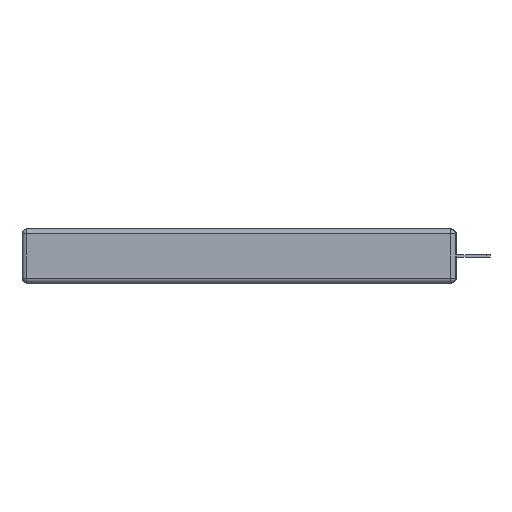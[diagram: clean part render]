
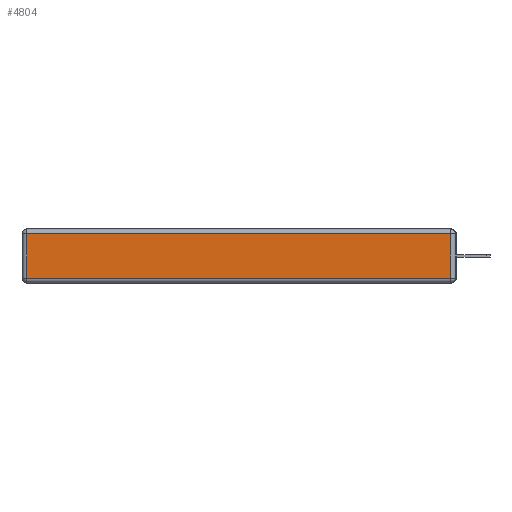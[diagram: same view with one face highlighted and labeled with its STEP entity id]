
A CAD part, left-side view. The second image highlights one B-rep face of the part: STEP entity #4804.
In plain terms, the highlighted planar face has unit normal (-1, 0, 0).
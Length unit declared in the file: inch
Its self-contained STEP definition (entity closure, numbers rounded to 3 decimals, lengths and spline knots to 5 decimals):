
#715 = EDGE_CURVE ( 'NONE', #19303, #4121, #13686, .T. ) ;
#1388 = VERTEX_POINT ( 'NONE', #10222 ) ;
#2633 = FACE_OUTER_BOUND ( 'NONE', #12897, .T. ) ;
#3143 = EDGE_CURVE ( 'NONE', #7421, #19303, #9139, .T. ) ;
#4050 = LINE ( 'NONE', #9018, #18800 ) ;
#4121 = VERTEX_POINT ( 'NONE', #5775 ) ;
#4445 = ORIENTED_EDGE ( 'NONE', *, *, #8056, .T. ) ;
#4685 = CARTESIAN_POINT ( 'NONE',  ( 0., 2.72, -0.343 ) ) ;
#4795 = VECTOR ( 'NONE', #10727, 39.37008 ) ;
#4801 = PLANE ( 'NONE',  #19844 ) ;
#4804 = ADVANCED_FACE ( 'NONE', ( #2633 ), #4801, .T. ) ;
#4899 = ORIENTED_EDGE ( 'NONE', *, *, #3143, .T. ) ;
#5522 = VECTOR ( 'NONE', #20512, 39.37008 ) ;
#5775 = CARTESIAN_POINT ( 'NONE',  ( 0., 0.03, -0.313 ) ) ;
#5783 = VECTOR ( 'NONE', #17182, 39.37008 ) ;
#7421 = VERTEX_POINT ( 'NONE', #14932 ) ;
#7989 = DIRECTION ( 'NONE',  ( -1., 0., 0. ) ) ;
#8056 = EDGE_CURVE ( 'NONE', #1388, #7421, #4050, .T. ) ;
#9018 = CARTESIAN_POINT ( 'NONE',  ( 0., 2.75, -0.03 ) ) ;
#9139 = LINE ( 'NONE', #4685, #4795 ) ;
#10222 = CARTESIAN_POINT ( 'NONE',  ( 0., 0.03, -0.03 ) ) ;
#10727 = DIRECTION ( 'NONE',  ( 0., 0., -1. ) ) ;
#12419 = DIRECTION ( 'NONE',  ( 0., 1., 0. ) ) ;
#12897 = EDGE_LOOP ( 'NONE', ( #15168, #16672, #4445, #4899 ) ) ;
#13451 = EDGE_CURVE ( 'NONE', #4121, #1388, #15949, .T. ) ;
#13686 = LINE ( 'NONE', #17479, #5783 ) ;
#14484 = CARTESIAN_POINT ( 'NONE',  ( 0., 0., -0.343 ) ) ;
#14932 = CARTESIAN_POINT ( 'NONE',  ( 0., 2.72, -0.03 ) ) ;
#15168 = ORIENTED_EDGE ( 'NONE', *, *, #715, .T. ) ;
#15809 = CARTESIAN_POINT ( 'NONE',  ( 0., 2.72, -0.313 ) ) ;
#15949 = LINE ( 'NONE', #18897, #5522 ) ;
#16672 = ORIENTED_EDGE ( 'NONE', *, *, #13451, .T. ) ;
#17182 = DIRECTION ( 'NONE',  ( 0., -1., 0. ) ) ;
#17479 = CARTESIAN_POINT ( 'NONE',  ( 0., 0., -0.313 ) ) ;
#18800 = VECTOR ( 'NONE', #12419, 39.37008 ) ;
#18897 = CARTESIAN_POINT ( 'NONE',  ( 0., 0.03, -0.343 ) ) ;
#19303 = VERTEX_POINT ( 'NONE', #15809 ) ;
#19330 = DIRECTION ( 'NONE',  ( 0., 0., 1. ) ) ;
#19844 = AXIS2_PLACEMENT_3D ( 'NONE', #14484, #7989, #19330 ) ;
#20512 = DIRECTION ( 'NONE',  ( 0., 0., 1. ) ) ;
